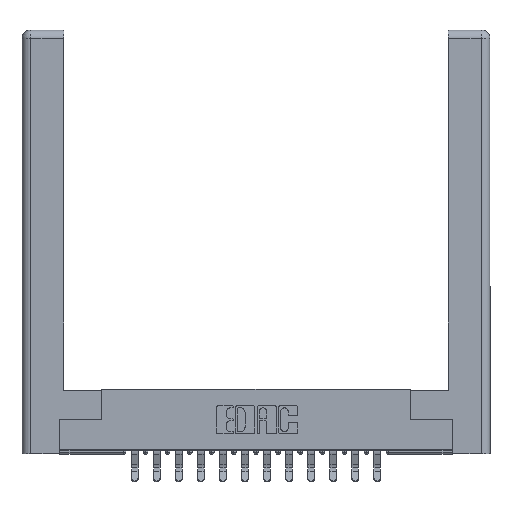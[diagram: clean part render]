
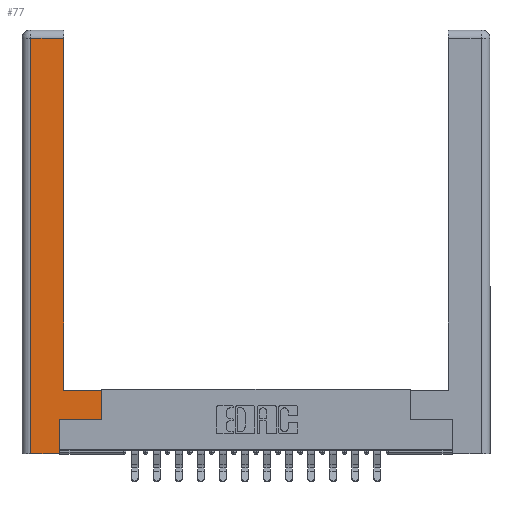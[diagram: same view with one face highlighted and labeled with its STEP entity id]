
A CAD part, top view. The second image highlights one B-rep face of the part: STEP entity #77.
In plain terms, the highlighted planar face has unit normal (0, 0, 1).
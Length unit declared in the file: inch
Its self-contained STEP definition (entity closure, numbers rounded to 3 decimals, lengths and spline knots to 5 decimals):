
#77 = ADVANCED_FACE ( 'NONE', ( #11270 ), #18137, .F. ) ;
#136 = EDGE_CURVE ( 'NONE', #8279, #11990, #12448, .T. ) ;
#1340 = VECTOR ( 'NONE', #10129, 39.37008 ) ;
#2362 = LINE ( 'NONE', #4321, #11601 ) ;
#2797 = VERTEX_POINT ( 'NONE', #4470 ) ;
#2812 = VECTOR ( 'NONE', #9197, 39.37008 ) ;
#2818 = VERTEX_POINT ( 'NONE', #6602 ) ;
#4029 = CARTESIAN_POINT ( 'NONE',  ( 0.295, 3., 0. ) ) ;
#4032 = EDGE_CURVE ( 'NONE', #2797, #12108, #2362, .T. ) ;
#4158 = DIRECTION ( 'NONE',  ( 1., 0., 0. ) ) ;
#4285 = CARTESIAN_POINT ( 'NONE',  ( 0.565, 0.245, 0. ) ) ;
#4321 = CARTESIAN_POINT ( 'NONE',  ( 0.565, 0.245, 0. ) ) ;
#4462 = EDGE_CURVE ( 'NONE', #5428, #2797, #12360, .T. ) ;
#4470 = CARTESIAN_POINT ( 'NONE',  ( 0.265, 0.245, 0. ) ) ;
#4580 = CARTESIAN_POINT ( 'NONE',  ( 0., 0., 0. ) ) ;
#4926 = ORIENTED_EDGE ( 'NONE', *, *, #4032, .T. ) ;
#5113 = VERTEX_POINT ( 'NONE', #14628 ) ;
#5165 = DIRECTION ( 'NONE',  ( 0., 1., 0. ) ) ;
#5428 = VERTEX_POINT ( 'NONE', #8502 ) ;
#6177 = ORIENTED_EDGE ( 'NONE', *, *, #13947, .T. ) ;
#6190 = DIRECTION ( 'NONE',  ( 0., 0., -1. ) ) ;
#6352 = CARTESIAN_POINT ( 'NONE',  ( 0.295, 2.94, 0. ) ) ;
#6602 = CARTESIAN_POINT ( 'NONE',  ( 0.565, 0.45, 0. ) ) ;
#7315 = EDGE_CURVE ( 'NONE', #12108, #2818, #10846, .T. ) ;
#7398 = CARTESIAN_POINT ( 'NONE',  ( 0.565, 0.45, 0. ) ) ;
#7918 = CARTESIAN_POINT ( 'NONE',  ( 0.0615, 2.94, 0. ) ) ;
#8049 = ORIENTED_EDGE ( 'NONE', *, *, #9994, .T. ) ;
#8279 = VERTEX_POINT ( 'NONE', #6352 ) ;
#8462 = ORIENTED_EDGE ( 'NONE', *, *, #8694, .T. ) ;
#8502 = CARTESIAN_POINT ( 'NONE',  ( 0.265, 0., 0. ) ) ;
#8694 = EDGE_CURVE ( 'NONE', #5113, #8279, #17873, .T. ) ;
#9107 = VERTEX_POINT ( 'NONE', #18872 ) ;
#9197 = DIRECTION ( 'NONE',  ( 0., 1., 0. ) ) ;
#9403 = CARTESIAN_POINT ( 'NONE',  ( 0.0615, 2.94, 0. ) ) ;
#9994 = EDGE_CURVE ( 'NONE', #9107, #5428, #10291, .T. ) ;
#9996 = ORIENTED_EDGE ( 'NONE', *, *, #7315, .T. ) ;
#10129 = DIRECTION ( 'NONE',  ( 0., 1., 0. ) ) ;
#10260 = LINE ( 'NONE', #12544, #12832 ) ;
#10291 = LINE ( 'NONE', #19136, #18514 ) ;
#10846 = LINE ( 'NONE', #7398, #2812 ) ;
#11180 = VECTOR ( 'NONE', #5165, 39.37008 ) ;
#11270 = FACE_OUTER_BOUND ( 'NONE', #15147, .T. ) ;
#11601 = VECTOR ( 'NONE', #17718, 39.37008 ) ;
#11745 = VECTOR ( 'NONE', #16171, 39.37008 ) ;
#11892 = AXIS2_PLACEMENT_3D ( 'NONE', #4580, #6190, #18265 ) ;
#11990 = VERTEX_POINT ( 'NONE', #9403 ) ;
#12108 = VERTEX_POINT ( 'NONE', #4285 ) ;
#12360 = LINE ( 'NONE', #14416, #11180 ) ;
#12448 = LINE ( 'NONE', #7918, #18573 ) ;
#12544 = CARTESIAN_POINT ( 'NONE',  ( 0.0615, 0., 0. ) ) ;
#12675 = DIRECTION ( 'NONE',  ( 0., -1., 0. ) ) ;
#12832 = VECTOR ( 'NONE', #12675, 39.37008 ) ;
#13947 = EDGE_CURVE ( 'NONE', #11990, #9107, #10260, .T. ) ;
#14416 = CARTESIAN_POINT ( 'NONE',  ( 0.265, 0.245, 0. ) ) ;
#14628 = CARTESIAN_POINT ( 'NONE',  ( 0.295, 0.45, 0. ) ) ;
#15147 = EDGE_LOOP ( 'NONE', ( #8462, #19148, #6177, #8049, #16387, #4926, #9996, #18801 ) ) ;
#15203 = DIRECTION ( 'NONE',  ( -1., 0., 0. ) ) ;
#15977 = CARTESIAN_POINT ( 'NONE',  ( 0.295, 0.45, 0. ) ) ;
#16171 = DIRECTION ( 'NONE',  ( -1., 0., 0. ) ) ;
#16387 = ORIENTED_EDGE ( 'NONE', *, *, #4462, .T. ) ;
#17181 = LINE ( 'NONE', #15977, #11745 ) ;
#17456 = EDGE_CURVE ( 'NONE', #2818, #5113, #17181, .T. ) ;
#17718 = DIRECTION ( 'NONE',  ( 1., 0., 0. ) ) ;
#17873 = LINE ( 'NONE', #4029, #1340 ) ;
#18137 = PLANE ( 'NONE',  #11892 ) ;
#18265 = DIRECTION ( 'NONE',  ( -1., 0., 0. ) ) ;
#18514 = VECTOR ( 'NONE', #4158, 39.37008 ) ;
#18573 = VECTOR ( 'NONE', #15203, 39.37008 ) ;
#18801 = ORIENTED_EDGE ( 'NONE', *, *, #17456, .T. ) ;
#18872 = CARTESIAN_POINT ( 'NONE',  ( 0.0615, 0., 0. ) ) ;
#19136 = CARTESIAN_POINT ( 'NONE',  ( 0.265, 0., 0. ) ) ;
#19148 = ORIENTED_EDGE ( 'NONE', *, *, #136, .T. ) ;
